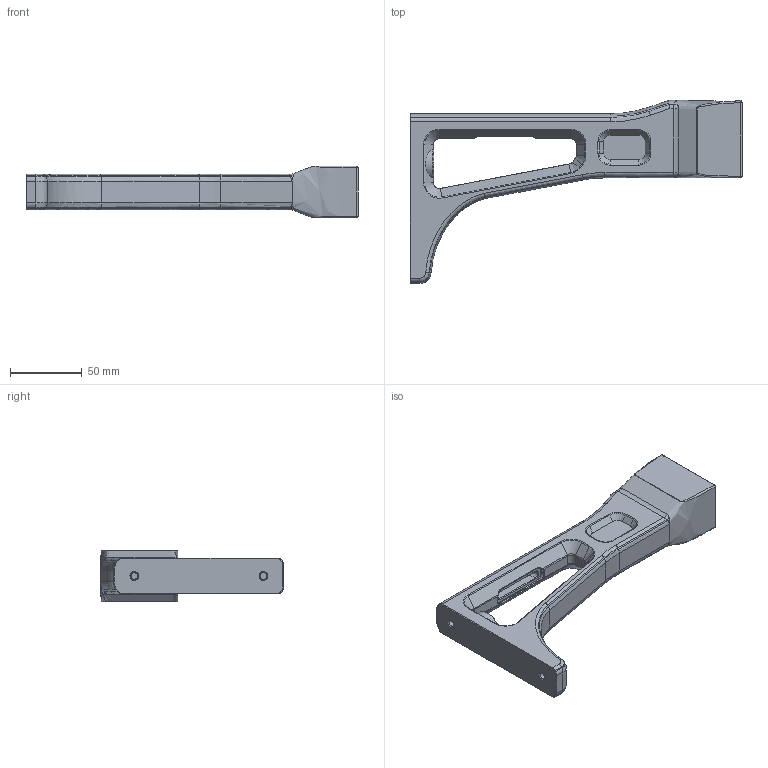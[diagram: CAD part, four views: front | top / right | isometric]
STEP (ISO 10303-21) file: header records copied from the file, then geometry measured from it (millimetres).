
FILE_DESCRIPTION (( 'STEP AP203' ), '1' );
FILE_NAME ('MOD9_G36_stock.STEP', '2020-07-07T01:44:46', ( '' ), ( '' ), 'SwSTEP 2.0', 'SolidWorks 2016', '' );
FILE_SCHEMA (( 'CONFIG_CONTROL_DESIGN' ));
Length unit declared in the file: millimetre
Products named in the file (1): MOD9_G36_stock
Bounding box: 231.4 x 127.58 x 36 mm (x, y, z)
Volume: 256211 mm3; surface area: 46129.4 mm2
Topology: 1 solids, 1 shells, 319 faces, 721 edges, 406 vertices
Faces by surface type: bspline 142, plane 87, cone 37, cylinder 35, torus 14, sphere 4
Full cylindrical faces by diameter (mm): 4.5 x2, 9.6 x1, 10 x1
Entity records: 15107 total; most frequent: CARTESIAN_POINT 9031, ORIENTED_EDGE 1408, DIRECTION 986, EDGE_CURVE 704, VERTEX_POINT 405, EDGE_LOOP 341, AXIS2_PLACEMENT_3D 329, LINE 328
